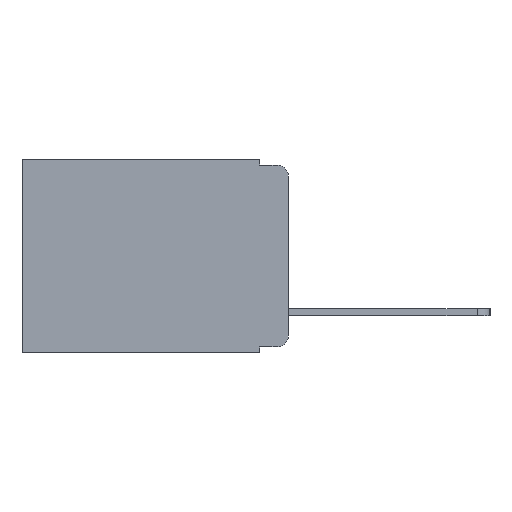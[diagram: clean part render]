
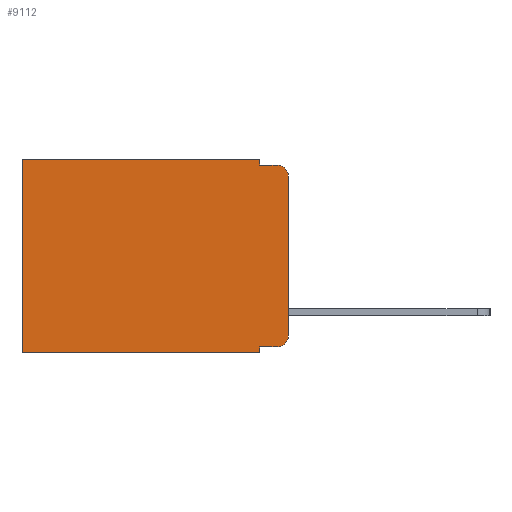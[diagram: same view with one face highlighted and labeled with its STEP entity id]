
A CAD part, left-side view. The second image highlights one B-rep face of the part: STEP entity #9112.
In plain terms, the highlighted planar face has unit normal (-1, 0, 0).
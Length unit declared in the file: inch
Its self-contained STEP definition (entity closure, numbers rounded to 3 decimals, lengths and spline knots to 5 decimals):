
#587 = EDGE_CURVE ( 'NONE', #14146, #1218, #16766, .T. ) ;
#615 = CARTESIAN_POINT ( 'NONE',  ( 0.298, 0.473, -0.343 ) ) ;
#632 = VERTEX_POINT ( 'NONE', #8369 ) ;
#803 = DIRECTION ( 'NONE',  ( 0., 0., -1. ) ) ;
#1116 = VECTOR ( 'NONE', #6166, 39.37008 ) ;
#1151 = ORIENTED_EDGE ( 'NONE', *, *, #587, .F. ) ;
#1218 = VERTEX_POINT ( 'NONE', #15408 ) ;
#1680 = EDGE_CURVE ( 'NONE', #4918, #17121, #18128, .T. ) ;
#1708 = VERTEX_POINT ( 'NONE', #4409 ) ;
#1762 = DIRECTION ( 'NONE',  ( -1., 0., 0. ) ) ;
#1903 = ORIENTED_EDGE ( 'NONE', *, *, #5945, .T. ) ;
#2398 = LINE ( 'NONE', #14956, #10372 ) ;
#2558 = DIRECTION ( 'NONE',  ( 1., 0., 0. ) ) ;
#2621 = EDGE_CURVE ( 'NONE', #1708, #4918, #5358, .T. ) ;
#2746 = EDGE_CURVE ( 'NONE', #1708, #4309, #11835, .T. ) ;
#2762 = CARTESIAN_POINT ( 'NONE',  ( 0.298, 0., 0. ) ) ;
#3208 = DIRECTION ( 'NONE',  ( 0., 0., -1. ) ) ;
#3763 = LINE ( 'NONE', #14906, #15308 ) ;
#3838 = CARTESIAN_POINT ( 'NONE',  ( 0.298, 0., 0. ) ) ;
#3986 = VERTEX_POINT ( 'NONE', #15856 ) ;
#3987 = CARTESIAN_POINT ( 'NONE',  ( 0.298, 0.051, -0.01 ) ) ;
#4192 = AXIS2_PLACEMENT_3D ( 'NONE', #12072, #2558, #13624 ) ;
#4309 = VERTEX_POINT ( 'NONE', #3987 ) ;
#4384 = ORIENTED_EDGE ( 'NONE', *, *, #10868, .F. ) ;
#4409 = CARTESIAN_POINT ( 'NONE',  ( 0.298, 0.051, 0. ) ) ;
#4451 = CIRCLE ( 'NONE', #13555, 0.02 ) ;
#4856 = EDGE_CURVE ( 'NONE', #4309, #3986, #3763, .T. ) ;
#4918 = VERTEX_POINT ( 'NONE', #5631 ) ;
#5358 = LINE ( 'NONE', #2762, #1116 ) ;
#5394 = ORIENTED_EDGE ( 'NONE', *, *, #19678, .T. ) ;
#5614 = DIRECTION ( 'NONE',  ( 0., 1., 0. ) ) ;
#5631 = CARTESIAN_POINT ( 'NONE',  ( 0.298, 0.473, 0. ) ) ;
#5642 = VECTOR ( 'NONE', #3208, 39.37008 ) ;
#5945 = EDGE_CURVE ( 'NONE', #17684, #3986, #4451, .T. ) ;
#6166 = DIRECTION ( 'NONE',  ( 0., 1., 0. ) ) ;
#6643 = LINE ( 'NONE', #3838, #5642 ) ;
#6795 = CARTESIAN_POINT ( 'NONE',  ( 0.298, 0.051, -0.333 ) ) ;
#7376 = DIRECTION ( 'NONE',  ( 0., -1., 0. ) ) ;
#8069 = EDGE_CURVE ( 'NONE', #17684, #12013, #6643, .T. ) ;
#8099 = CARTESIAN_POINT ( 'NONE',  ( 0.298, 0.02, -0.03 ) ) ;
#8369 = CARTESIAN_POINT ( 'NONE',  ( 0.298, 0.02, -0.333 ) ) ;
#8433 = VECTOR ( 'NONE', #7376, 39.37008 ) ;
#8854 = DIRECTION ( 'NONE',  ( 0., -1., 0. ) ) ;
#9112 = ADVANCED_FACE ( 'NONE', ( #13634 ), #11946, .F. ) ;
#9670 = EDGE_LOOP ( 'NONE', ( #17967, #1903, #14493, #15423, #11868, #16369, #4384, #1151, #5394, #14263 ) ) ;
#10047 = VECTOR ( 'NONE', #19323, 39.37008 ) ;
#10077 = CARTESIAN_POINT ( 'NONE',  ( 0.298, 0., -0.03 ) ) ;
#10317 = AXIS2_PLACEMENT_3D ( 'NONE', #11296, #1762, #12854 ) ;
#10372 = VECTOR ( 'NONE', #5614, 39.37008 ) ;
#10868 = EDGE_CURVE ( 'NONE', #1218, #17121, #2398, .T. ) ;
#11021 = CARTESIAN_POINT ( 'NONE',  ( 0.298, 0.473, 0. ) ) ;
#11296 = CARTESIAN_POINT ( 'NONE',  ( 0.298, 0.02, -0.313 ) ) ;
#11603 = CARTESIAN_POINT ( 'NONE',  ( 0.298, 0.051, 0. ) ) ;
#11835 = LINE ( 'NONE', #11603, #14935 ) ;
#11868 = ORIENTED_EDGE ( 'NONE', *, *, #2621, .T. ) ;
#11946 = PLANE ( 'NONE',  #4192 ) ;
#12013 = VERTEX_POINT ( 'NONE', #19011 ) ;
#12072 = CARTESIAN_POINT ( 'NONE',  ( 0.298, 0., 0. ) ) ;
#12142 = LINE ( 'NONE', #16652, #8433 ) ;
#12743 = CARTESIAN_POINT ( 'NONE',  ( 0.298, 0.051, 0. ) ) ;
#12854 = DIRECTION ( 'NONE',  ( 0., 0., -1. ) ) ;
#13555 = AXIS2_PLACEMENT_3D ( 'NONE', #8099, #18799, #15968 ) ;
#13624 = DIRECTION ( 'NONE',  ( 0., 0., -1. ) ) ;
#13634 = FACE_OUTER_BOUND ( 'NONE', #9670, .T. ) ;
#14146 = VERTEX_POINT ( 'NONE', #6795 ) ;
#14263 = ORIENTED_EDGE ( 'NONE', *, *, #18700, .T. ) ;
#14493 = ORIENTED_EDGE ( 'NONE', *, *, #4856, .F. ) ;
#14906 = CARTESIAN_POINT ( 'NONE',  ( 0.298, 0.051, -0.01 ) ) ;
#14935 = VECTOR ( 'NONE', #803, 39.37008 ) ;
#14956 = CARTESIAN_POINT ( 'NONE',  ( 0.298, 0., -0.343 ) ) ;
#15308 = VECTOR ( 'NONE', #8854, 39.37008 ) ;
#15408 = CARTESIAN_POINT ( 'NONE',  ( 0.298, 0.051, -0.343 ) ) ;
#15423 = ORIENTED_EDGE ( 'NONE', *, *, #2746, .F. ) ;
#15856 = CARTESIAN_POINT ( 'NONE',  ( 0.298, 0.02, -0.01 ) ) ;
#15968 = DIRECTION ( 'NONE',  ( 0., 0., -1. ) ) ;
#16309 = VECTOR ( 'NONE', #18465, 39.37008 ) ;
#16369 = ORIENTED_EDGE ( 'NONE', *, *, #1680, .T. ) ;
#16652 = CARTESIAN_POINT ( 'NONE',  ( 0.298, 0.051, -0.333 ) ) ;
#16766 = LINE ( 'NONE', #12743, #16309 ) ;
#17121 = VERTEX_POINT ( 'NONE', #615 ) ;
#17684 = VERTEX_POINT ( 'NONE', #10077 ) ;
#17967 = ORIENTED_EDGE ( 'NONE', *, *, #8069, .F. ) ;
#18128 = LINE ( 'NONE', #11021, #10047 ) ;
#18465 = DIRECTION ( 'NONE',  ( 0., 0., -1. ) ) ;
#18514 = CIRCLE ( 'NONE', #10317, 0.02 ) ;
#18700 = EDGE_CURVE ( 'NONE', #632, #12013, #18514, .T. ) ;
#18799 = DIRECTION ( 'NONE',  ( -1., 0., 0. ) ) ;
#19011 = CARTESIAN_POINT ( 'NONE',  ( 0.298, 0., -0.313 ) ) ;
#19323 = DIRECTION ( 'NONE',  ( 0., 0., -1. ) ) ;
#19678 = EDGE_CURVE ( 'NONE', #14146, #632, #12142, .T. ) ;
